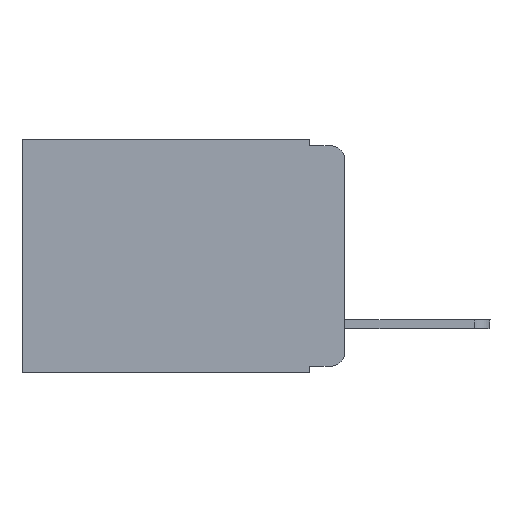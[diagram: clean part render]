
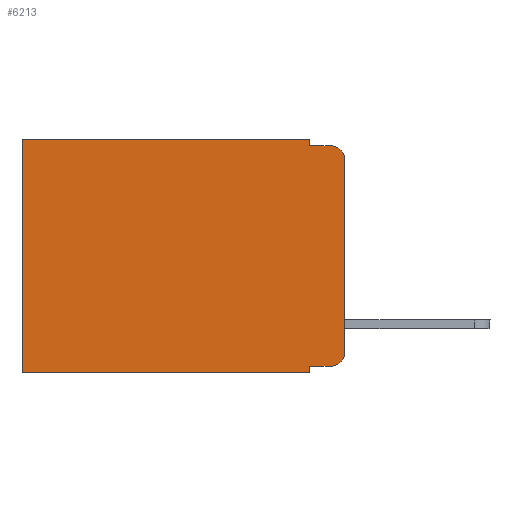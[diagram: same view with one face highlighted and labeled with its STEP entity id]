
A CAD part, left-side view. The second image highlights one B-rep face of the part: STEP entity #6213.
In plain terms, the highlighted planar face has unit normal (-1, 0, 0).
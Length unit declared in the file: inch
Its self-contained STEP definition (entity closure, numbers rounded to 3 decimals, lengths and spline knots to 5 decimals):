
#91 = VECTOR ( 'NONE', #6643, 39.37008 ) ;
#389 = VERTEX_POINT ( 'NONE', #6978 ) ;
#441 = LINE ( 'NONE', #7754, #91 ) ;
#586 = CARTESIAN_POINT ( 'NONE',  ( 0.298, 0.051, 0. ) ) ;
#811 = DIRECTION ( 'NONE',  ( 1., 0., 0. ) ) ;
#976 = EDGE_CURVE ( 'NONE', #1438, #13915, #14896, .T. ) ;
#1248 = AXIS2_PLACEMENT_3D ( 'NONE', #9145, #2284, #11663 ) ;
#1282 = ORIENTED_EDGE ( 'NONE', *, *, #5941, .T. ) ;
#1403 = CARTESIAN_POINT ( 'NONE',  ( 0.298, 0.051, -0.343 ) ) ;
#1438 = VERTEX_POINT ( 'NONE', #7925 ) ;
#1617 = ORIENTED_EDGE ( 'NONE', *, *, #10346, .F. ) ;
#1650 = DIRECTION ( 'NONE',  ( 0., 0., -1. ) ) ;
#1870 = CARTESIAN_POINT ( 'NONE',  ( 0.298, 0.473, -0.343 ) ) ;
#1946 = DIRECTION ( 'NONE',  ( 0., 1., 0. ) ) ;
#1950 = VECTOR ( 'NONE', #2676, 39.37008 ) ;
#2066 = CARTESIAN_POINT ( 'NONE',  ( 0.298, 0.02, -0.03 ) ) ;
#2171 = VERTEX_POINT ( 'NONE', #1870 ) ;
#2284 = DIRECTION ( 'NONE',  ( -1., 0., 0. ) ) ;
#2324 = VERTEX_POINT ( 'NONE', #14640 ) ;
#2535 = VECTOR ( 'NONE', #7217, 39.37008 ) ;
#2672 = DIRECTION ( 'NONE',  ( 0., 0., -1. ) ) ;
#2676 = DIRECTION ( 'NONE',  ( 0., 1., 0. ) ) ;
#2793 = DIRECTION ( 'NONE',  ( 0., -1., 0. ) ) ;
#2991 = LINE ( 'NONE', #5740, #6279 ) ;
#3333 = DIRECTION ( 'NONE',  ( -1., 0., 0. ) ) ;
#3590 = VECTOR ( 'NONE', #1946, 39.37008 ) ;
#3806 = VERTEX_POINT ( 'NONE', #5657 ) ;
#4446 = DIRECTION ( 'NONE',  ( 0., 0., -1. ) ) ;
#4675 = LINE ( 'NONE', #14536, #8341 ) ;
#4676 = ORIENTED_EDGE ( 'NONE', *, *, #14582, .T. ) ;
#4868 = CARTESIAN_POINT ( 'NONE',  ( 0.298, 0.473, 0. ) ) ;
#4918 = ORIENTED_EDGE ( 'NONE', *, *, #976, .T. ) ;
#5087 = EDGE_CURVE ( 'NONE', #389, #7275, #11868, .T. ) ;
#5431 = CARTESIAN_POINT ( 'NONE',  ( 0.298, 0., 0. ) ) ;
#5657 = CARTESIAN_POINT ( 'NONE',  ( 0.298, 0.051, -0.333 ) ) ;
#5663 = AXIS2_PLACEMENT_3D ( 'NONE', #5431, #811, #13664 ) ;
#5740 = CARTESIAN_POINT ( 'NONE',  ( 0.298, 0.051, -0.333 ) ) ;
#5941 = EDGE_CURVE ( 'NONE', #13988, #2324, #5972, .T. ) ;
#5972 = LINE ( 'NONE', #9683, #1950 ) ;
#6213 = ADVANCED_FACE ( 'NONE', ( #13111 ), #7783, .F. ) ;
#6233 = EDGE_LOOP ( 'NONE', ( #11704, #4918, #1617, #8639, #1282, #4676, #10458, #6716, #12539, #6496 ) ) ;
#6279 = VECTOR ( 'NONE', #8033, 39.37008 ) ;
#6496 = ORIENTED_EDGE ( 'NONE', *, *, #5087, .T. ) ;
#6643 = DIRECTION ( 'NONE',  ( 0., 0., -1. ) ) ;
#6716 = ORIENTED_EDGE ( 'NONE', *, *, #14736, .F. ) ;
#6739 = EDGE_CURVE ( 'NONE', #3806, #389, #2991, .T. ) ;
#6867 = VERTEX_POINT ( 'NONE', #1403 ) ;
#6978 = CARTESIAN_POINT ( 'NONE',  ( 0.298, 0.02, -0.333 ) ) ;
#7039 = EDGE_CURVE ( 'NONE', #13988, #14763, #13096, .T. ) ;
#7148 = CARTESIAN_POINT ( 'NONE',  ( 0.298, 0., -0.313 ) ) ;
#7217 = DIRECTION ( 'NONE',  ( 0., 0., -1. ) ) ;
#7275 = VERTEX_POINT ( 'NONE', #7148 ) ;
#7662 = EDGE_CURVE ( 'NONE', #1438, #7275, #441, .T. ) ;
#7754 = CARTESIAN_POINT ( 'NONE',  ( 0.298, 0., 0. ) ) ;
#7783 = PLANE ( 'NONE',  #5663 ) ;
#7925 = CARTESIAN_POINT ( 'NONE',  ( 0.298, 0., -0.03 ) ) ;
#8033 = DIRECTION ( 'NONE',  ( 0., -1., 0. ) ) ;
#8341 = VECTOR ( 'NONE', #2793, 39.37008 ) ;
#8639 = ORIENTED_EDGE ( 'NONE', *, *, #7039, .F. ) ;
#8755 = LINE ( 'NONE', #4868, #2535 ) ;
#8941 = LINE ( 'NONE', #14407, #14824 ) ;
#9112 = CARTESIAN_POINT ( 'NONE',  ( 0.298, 0.051, 0. ) ) ;
#9145 = CARTESIAN_POINT ( 'NONE',  ( 0.298, 0.02, -0.313 ) ) ;
#9683 = CARTESIAN_POINT ( 'NONE',  ( 0.298, 0., 0. ) ) ;
#9698 = EDGE_CURVE ( 'NONE', #6867, #2171, #9984, .T. ) ;
#9942 = VECTOR ( 'NONE', #1650, 39.37008 ) ;
#9984 = LINE ( 'NONE', #11366, #3590 ) ;
#10346 = EDGE_CURVE ( 'NONE', #14763, #13915, #4675, .T. ) ;
#10458 = ORIENTED_EDGE ( 'NONE', *, *, #9698, .F. ) ;
#11366 = CARTESIAN_POINT ( 'NONE',  ( 0.298, 0., -0.343 ) ) ;
#11663 = DIRECTION ( 'NONE',  ( 0., 0., -1. ) ) ;
#11704 = ORIENTED_EDGE ( 'NONE', *, *, #7662, .F. ) ;
#11868 = CIRCLE ( 'NONE', #1248, 0.02 ) ;
#11896 = AXIS2_PLACEMENT_3D ( 'NONE', #2066, #3333, #4446 ) ;
#12539 = ORIENTED_EDGE ( 'NONE', *, *, #6739, .T. ) ;
#13096 = LINE ( 'NONE', #586, #9942 ) ;
#13111 = FACE_OUTER_BOUND ( 'NONE', #6233, .T. ) ;
#13339 = CARTESIAN_POINT ( 'NONE',  ( 0.298, 0.051, -0.01 ) ) ;
#13664 = DIRECTION ( 'NONE',  ( 0., 0., -1. ) ) ;
#13794 = CARTESIAN_POINT ( 'NONE',  ( 0.298, 0.02, -0.01 ) ) ;
#13915 = VERTEX_POINT ( 'NONE', #13794 ) ;
#13988 = VERTEX_POINT ( 'NONE', #9112 ) ;
#14407 = CARTESIAN_POINT ( 'NONE',  ( 0.298, 0.051, 0. ) ) ;
#14536 = CARTESIAN_POINT ( 'NONE',  ( 0.298, 0.051, -0.01 ) ) ;
#14582 = EDGE_CURVE ( 'NONE', #2324, #2171, #8755, .T. ) ;
#14640 = CARTESIAN_POINT ( 'NONE',  ( 0.298, 0.473, 0. ) ) ;
#14736 = EDGE_CURVE ( 'NONE', #3806, #6867, #8941, .T. ) ;
#14763 = VERTEX_POINT ( 'NONE', #13339 ) ;
#14824 = VECTOR ( 'NONE', #2672, 39.37008 ) ;
#14896 = CIRCLE ( 'NONE', #11896, 0.02 ) ;
